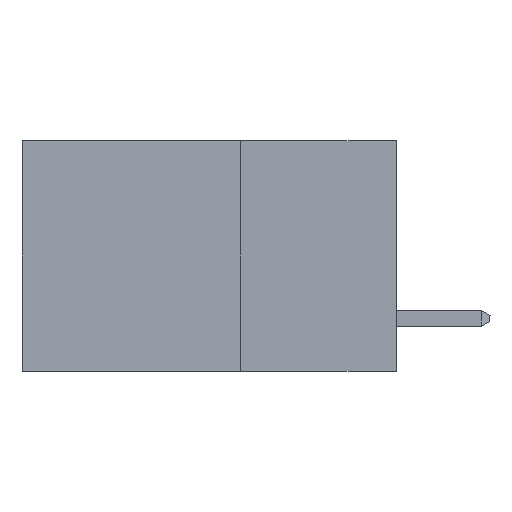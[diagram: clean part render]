
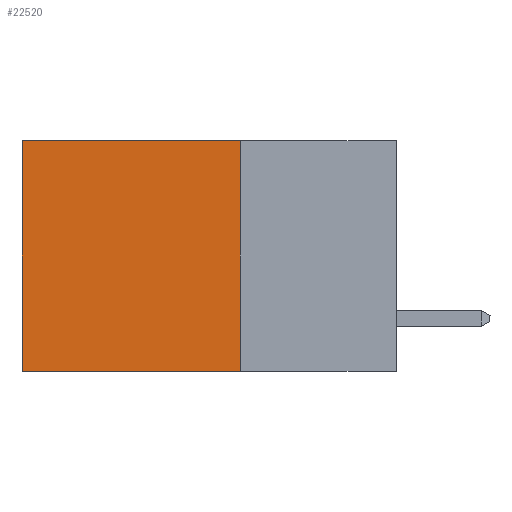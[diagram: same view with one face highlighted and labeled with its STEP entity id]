
A CAD part, left-side view. The second image highlights one B-rep face of the part: STEP entity #22520.
In plain terms, the highlighted planar face has unit normal (-1, 0, 0).
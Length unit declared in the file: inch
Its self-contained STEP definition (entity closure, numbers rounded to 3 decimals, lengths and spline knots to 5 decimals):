
#683 = LINE ( 'NONE', #21581, #25552 ) ;
#1067 = VERTEX_POINT ( 'NONE', #10435 ) ;
#2085 = ORIENTED_EDGE ( 'NONE', *, *, #27094, .F. ) ;
#3884 = LINE ( 'NONE', #17413, #22743 ) ;
#4681 = VECTOR ( 'NONE', #18232, 39.37008 ) ;
#5570 = CARTESIAN_POINT ( 'NONE',  ( 0.298, 0.6, 0. ) ) ;
#5691 = CARTESIAN_POINT ( 'NONE',  ( 0.298, 0.6, 0. ) ) ;
#6896 = CARTESIAN_POINT ( 'NONE',  ( 0.298, 0.25, 0. ) ) ;
#7150 = DIRECTION ( 'NONE',  ( 0., 1., 0. ) ) ;
#8759 = VECTOR ( 'NONE', #30600, 39.37008 ) ;
#10435 = CARTESIAN_POINT ( 'NONE',  ( 0.298, 0.6, -0.37 ) ) ;
#11129 = LINE ( 'NONE', #5691, #4681 ) ;
#11589 = DIRECTION ( 'NONE',  ( 1., 0., 0. ) ) ;
#11809 = DIRECTION ( 'NONE',  ( 0., 0., -1. ) ) ;
#16503 = PLANE ( 'NONE',  #22492 ) ;
#17169 = CARTESIAN_POINT ( 'NONE',  ( 0.298, 0.25, 0. ) ) ;
#17413 = CARTESIAN_POINT ( 'NONE',  ( 0.298, 0.25, 0. ) ) ;
#17480 = EDGE_CURVE ( 'NONE', #29616, #1067, #11129, .T. ) ;
#17896 = VERTEX_POINT ( 'NONE', #17169 ) ;
#18232 = DIRECTION ( 'NONE',  ( 0., 0., -1. ) ) ;
#19403 = DIRECTION ( 'NONE',  ( 0., 0., -1. ) ) ;
#21053 = CARTESIAN_POINT ( 'NONE',  ( 0.298, 0.25, -0.37 ) ) ;
#21581 = CARTESIAN_POINT ( 'NONE',  ( 0.298, 0.25, 0. ) ) ;
#22492 = AXIS2_PLACEMENT_3D ( 'NONE', #6896, #11589, #11809 ) ;
#22520 = ADVANCED_FACE ( 'NONE', ( #25157 ), #16503, .F. ) ;
#22743 = VECTOR ( 'NONE', #19403, 39.37008 ) ;
#23272 = CARTESIAN_POINT ( 'NONE',  ( 0.298, 0.25, -0.37 ) ) ;
#24221 = EDGE_LOOP ( 'NONE', ( #29027, #2085, #29370, #26627 ) ) ;
#25157 = FACE_OUTER_BOUND ( 'NONE', #24221, .T. ) ;
#25552 = VECTOR ( 'NONE', #7150, 39.37008 ) ;
#26627 = ORIENTED_EDGE ( 'NONE', *, *, #29968, .T. ) ;
#26705 = EDGE_CURVE ( 'NONE', #17896, #27093, #3884, .T. ) ;
#27093 = VERTEX_POINT ( 'NONE', #21053 ) ;
#27094 = EDGE_CURVE ( 'NONE', #27093, #1067, #30977, .T. ) ;
#29027 = ORIENTED_EDGE ( 'NONE', *, *, #17480, .T. ) ;
#29370 = ORIENTED_EDGE ( 'NONE', *, *, #26705, .F. ) ;
#29616 = VERTEX_POINT ( 'NONE', #5570 ) ;
#29968 = EDGE_CURVE ( 'NONE', #17896, #29616, #683, .T. ) ;
#30600 = DIRECTION ( 'NONE',  ( 0., 1., 0. ) ) ;
#30977 = LINE ( 'NONE', #23272, #8759 ) ;
